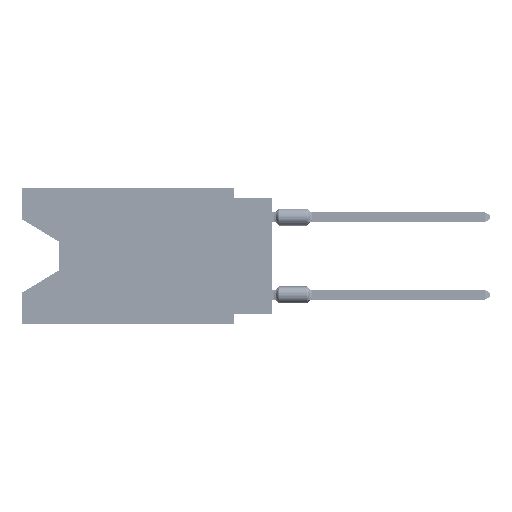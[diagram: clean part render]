
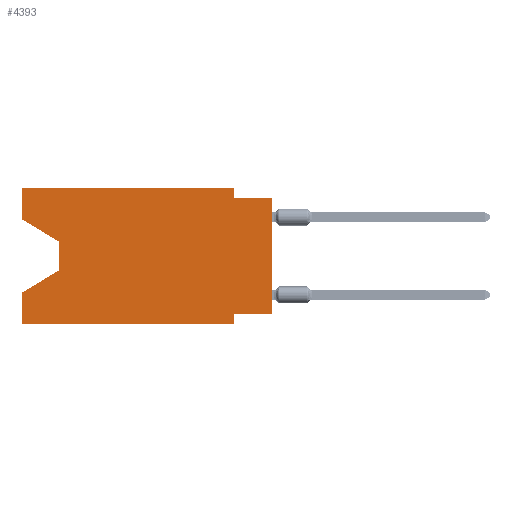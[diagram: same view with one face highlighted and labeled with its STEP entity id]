
A CAD part, left-side view. The second image highlights one B-rep face of the part: STEP entity #4393.
In plain terms, the highlighted planar face has unit normal (-1, 0, 0).
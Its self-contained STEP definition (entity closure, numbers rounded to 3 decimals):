
#1948 = EDGE_CURVE ( 'NONE', #36008, #22177, #10317, .T. ) ;
#2163 = CARTESIAN_POINT ( 'NONE',  ( 0., 16.383, 0. ) ) ;
#2831 = DIRECTION ( 'NONE',  ( 0., 0., 1. ) ) ;
#4393 = ADVANCED_FACE ( 'NONE', ( #6503 ), #63331, .F. ) ;
#4550 = EDGE_CURVE ( 'NONE', #70615, #62823, #25916, .T. ) ;
#4578 = CARTESIAN_POINT ( 'NONE',  ( 0., 16.383, -8.89 ) ) ;
#5132 = VECTOR ( 'NONE', #59117, 1000. ) ;
#5725 = CARTESIAN_POINT ( 'NONE',  ( 0., 2.54, -8.89 ) ) ;
#6381 = CARTESIAN_POINT ( 'NONE',  ( 0., 16.383, -6.852 ) ) ;
#6503 = FACE_OUTER_BOUND ( 'NONE', #19112, .T. ) ;
#7235 = LINE ( 'NONE', #36998, #21713 ) ;
#9579 = CARTESIAN_POINT ( 'NONE',  ( 0., 0., -8.255 ) ) ;
#9957 = VECTOR ( 'NONE', #40648, 1000. ) ;
#10139 = EDGE_CURVE ( 'NONE', #36263, #22177, #14541, .T. ) ;
#10186 = DIRECTION ( 'NONE',  ( 0., 0., -1. ) ) ;
#10317 = LINE ( 'NONE', #5725, #24342 ) ;
#11529 = DIRECTION ( 'NONE',  ( 0., 1., 0. ) ) ;
#12477 = DIRECTION ( 'NONE',  ( 0., 0., 1. ) ) ;
#12597 = CARTESIAN_POINT ( 'NONE',  ( 0., 13.97, -5.385 ) ) ;
#13528 = LINE ( 'NONE', #65369, #46684 ) ;
#13854 = CARTESIAN_POINT ( 'NONE',  ( 0., 2.54, 0. ) ) ;
#14009 = LINE ( 'NONE', #2163, #36072 ) ;
#14178 = DIRECTION ( 'NONE',  ( 0., -1., 0. ) ) ;
#14541 = LINE ( 'NONE', #32459, #31335 ) ;
#17316 = AXIS2_PLACEMENT_3D ( 'NONE', #41212, #46561, #29767 ) ;
#18378 = VECTOR ( 'NONE', #43076, 1000. ) ;
#19112 = EDGE_LOOP ( 'NONE', ( #23410, #64107, #25395, #42668, #33652, #70903, #47527, #32304, #69612, #41749, #39610, #26202 ) ) ;
#19783 = CARTESIAN_POINT ( 'NONE',  ( 0., 16.383, 0. ) ) ;
#21222 = EDGE_CURVE ( 'NONE', #63912, #36008, #57295, .T. ) ;
#21713 = VECTOR ( 'NONE', #25914, 1000. ) ;
#22177 = VERTEX_POINT ( 'NONE', #31440 ) ;
#23084 = LINE ( 'NONE', #46362, #9957 ) ;
#23410 = ORIENTED_EDGE ( 'NONE', *, *, #64576, .T. ) ;
#24231 = EDGE_CURVE ( 'NONE', #62887, #70615, #7235, .T. ) ;
#24342 = VECTOR ( 'NONE', #33961, 1000. ) ;
#25395 = ORIENTED_EDGE ( 'NONE', *, *, #4550, .T. ) ;
#25914 = DIRECTION ( 'NONE',  ( 0., 0., -1. ) ) ;
#25916 = LINE ( 'NONE', #12597, #5132 ) ;
#26202 = ORIENTED_EDGE ( 'NONE', *, *, #65312, .F. ) ;
#28442 = EDGE_CURVE ( 'NONE', #66229, #37103, #72015, .T. ) ;
#28847 = LINE ( 'NONE', #68145, #29617 ) ;
#29617 = VECTOR ( 'NONE', #10186, 1000. ) ;
#29767 = DIRECTION ( 'NONE',  ( 0., 0., -1. ) ) ;
#31335 = VECTOR ( 'NONE', #14178, 1000. ) ;
#31440 = CARTESIAN_POINT ( 'NONE',  ( 0., 2.54, -8.89 ) ) ;
#32012 = VERTEX_POINT ( 'NONE', #49978 ) ;
#32304 = ORIENTED_EDGE ( 'NONE', *, *, #66993, .T. ) ;
#32459 = CARTESIAN_POINT ( 'NONE',  ( 0., 16.383, -8.89 ) ) ;
#33652 = ORIENTED_EDGE ( 'NONE', *, *, #10139, .T. ) ;
#33961 = DIRECTION ( 'NONE',  ( 0., 0., -1. ) ) ;
#33982 = CARTESIAN_POINT ( 'NONE',  ( 0., 0., -0.635 ) ) ;
#35819 = CARTESIAN_POINT ( 'NONE',  ( 0., 2.54, -0.635 ) ) ;
#36008 = VERTEX_POINT ( 'NONE', #53065 ) ;
#36072 = VECTOR ( 'NONE', #12477, 1000. ) ;
#36263 = VERTEX_POINT ( 'NONE', #4578 ) ;
#36300 = CARTESIAN_POINT ( 'NONE',  ( 0., 16.383, 0. ) ) ;
#36881 = VERTEX_POINT ( 'NONE', #50884 ) ;
#36998 = CARTESIAN_POINT ( 'NONE',  ( 0., 13.97, -3.505 ) ) ;
#37103 = VERTEX_POINT ( 'NONE', #13854 ) ;
#39610 = ORIENTED_EDGE ( 'NONE', *, *, #28442, .F. ) ;
#40648 = DIRECTION ( 'NONE',  ( 0., -0.855, -0.519 ) ) ;
#41212 = CARTESIAN_POINT ( 'NONE',  ( 0., 16.383, 0. ) ) ;
#41749 = ORIENTED_EDGE ( 'NONE', *, *, #42923, .F. ) ;
#42668 = ORIENTED_EDGE ( 'NONE', *, *, #57949, .F. ) ;
#42923 = EDGE_CURVE ( 'NONE', #37103, #61428, #28847, .T. ) ;
#43076 = DIRECTION ( 'NONE',  ( 0., -1., 0. ) ) ;
#44304 = DIRECTION ( 'NONE',  ( 0., -1., 0. ) ) ;
#45810 = LINE ( 'NONE', #33982, #68811 ) ;
#46279 = CARTESIAN_POINT ( 'NONE',  ( 0., 13.97, -5.385 ) ) ;
#46362 = CARTESIAN_POINT ( 'NONE',  ( 0., 16.383, -2.038 ) ) ;
#46561 = DIRECTION ( 'NONE',  ( 1., 0., 0. ) ) ;
#46684 = VECTOR ( 'NONE', #2831, 1000. ) ;
#47527 = ORIENTED_EDGE ( 'NONE', *, *, #21222, .F. ) ;
#49978 = CARTESIAN_POINT ( 'NONE',  ( 0., 0., -0.635 ) ) ;
#50884 = CARTESIAN_POINT ( 'NONE',  ( 0., 16.383, -2.038 ) ) ;
#53065 = CARTESIAN_POINT ( 'NONE',  ( 0., 2.54, -8.255 ) ) ;
#53627 = DIRECTION ( 'NONE',  ( 0., 0., 1. ) ) ;
#57295 = LINE ( 'NONE', #64502, #70150 ) ;
#57871 = CARTESIAN_POINT ( 'NONE',  ( 0., 13.97, -3.505 ) ) ;
#57949 = EDGE_CURVE ( 'NONE', #36263, #62823, #14009, .T. ) ;
#59117 = DIRECTION ( 'NONE',  ( 0., 0.855, -0.519 ) ) ;
#61428 = VERTEX_POINT ( 'NONE', #35819 ) ;
#62823 = VERTEX_POINT ( 'NONE', #6381 ) ;
#62887 = VERTEX_POINT ( 'NONE', #57871 ) ;
#63331 = PLANE ( 'NONE',  #17316 ) ;
#63912 = VERTEX_POINT ( 'NONE', #9579 ) ;
#64107 = ORIENTED_EDGE ( 'NONE', *, *, #24231, .T. ) ;
#64502 = CARTESIAN_POINT ( 'NONE',  ( 0., 0., -8.255 ) ) ;
#64576 = EDGE_CURVE ( 'NONE', #36881, #62887, #23084, .T. ) ;
#65312 = EDGE_CURVE ( 'NONE', #36881, #66229, #65442, .T. ) ;
#65369 = CARTESIAN_POINT ( 'NONE',  ( 0., 0., 0. ) ) ;
#65442 = LINE ( 'NONE', #72291, #72101 ) ;
#66229 = VERTEX_POINT ( 'NONE', #36300 ) ;
#66993 = EDGE_CURVE ( 'NONE', #63912, #32012, #13528, .T. ) ;
#68145 = CARTESIAN_POINT ( 'NONE',  ( 0., 2.54, 0. ) ) ;
#68811 = VECTOR ( 'NONE', #44304, 1000. ) ;
#69147 = EDGE_CURVE ( 'NONE', #61428, #32012, #45810, .T. ) ;
#69612 = ORIENTED_EDGE ( 'NONE', *, *, #69147, .F. ) ;
#70150 = VECTOR ( 'NONE', #11529, 1000. ) ;
#70615 = VERTEX_POINT ( 'NONE', #46279 ) ;
#70903 = ORIENTED_EDGE ( 'NONE', *, *, #1948, .F. ) ;
#72015 = LINE ( 'NONE', #19783, #18378 ) ;
#72101 = VECTOR ( 'NONE', #53627, 1000. ) ;
#72291 = CARTESIAN_POINT ( 'NONE',  ( 0., 16.383, 0. ) ) ;
